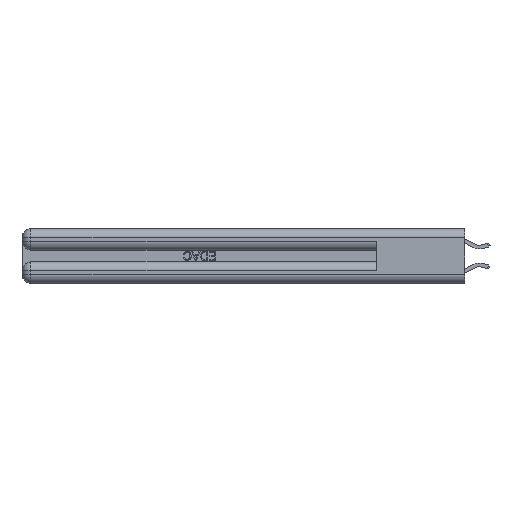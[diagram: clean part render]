
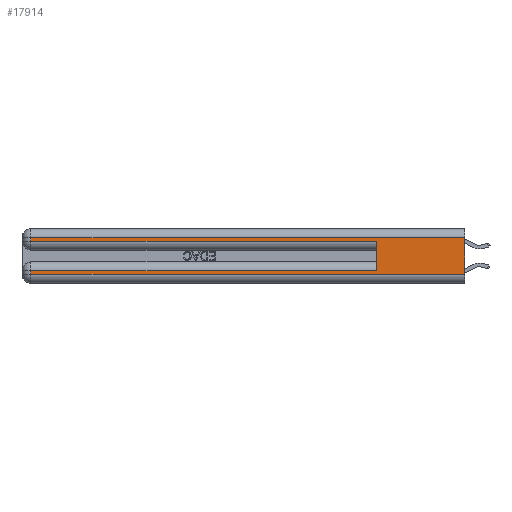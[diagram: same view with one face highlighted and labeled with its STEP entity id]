
A CAD part, left-side view. The second image highlights one B-rep face of the part: STEP entity #17914.
In plain terms, the highlighted planar face has unit normal (-1, 0, 0).
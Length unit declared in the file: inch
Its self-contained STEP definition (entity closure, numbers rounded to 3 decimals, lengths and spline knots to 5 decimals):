
#242 = VERTEX_POINT ( 'NONE', #15075 ) ;
#942 = CARTESIAN_POINT ( 'NONE',  ( 0., 0., 0.06 ) ) ;
#944 = EDGE_CURVE ( 'NONE', #242, #6256, #5850, .T. ) ;
#1041 = FACE_OUTER_BOUND ( 'NONE', #23048, .T. ) ;
#1250 = PLANE ( 'NONE',  #2903 ) ;
#1401 = CARTESIAN_POINT ( 'NONE',  ( 0., 0., 0.37 ) ) ;
#1502 = EDGE_CURVE ( 'NONE', #28715, #6095, #22812, .T. ) ;
#2055 = LINE ( 'NONE', #942, #10357 ) ;
#2480 = CARTESIAN_POINT ( 'NONE',  ( 0., 0.6, 0.285 ) ) ;
#2903 = AXIS2_PLACEMENT_3D ( 'NONE', #13322, #5729, #13222 ) ;
#3819 = DIRECTION ( 'NONE',  ( 0., -1., 0. ) ) ;
#4041 = VECTOR ( 'NONE', #26148, 39.37008 ) ;
#4274 = VERTEX_POINT ( 'NONE', #15329 ) ;
#5330 = CARTESIAN_POINT ( 'NONE',  ( 0., 2.94, 0.37 ) ) ;
#5620 = VECTOR ( 'NONE', #29505, 39.37008 ) ;
#5729 = DIRECTION ( 'NONE',  ( 1., 0., 0. ) ) ;
#5850 = LINE ( 'NONE', #30965, #7732 ) ;
#6095 = VERTEX_POINT ( 'NONE', #23312 ) ;
#6256 = VERTEX_POINT ( 'NONE', #2480 ) ;
#6715 = LINE ( 'NONE', #16120, #9333 ) ;
#6733 = ORIENTED_EDGE ( 'NONE', *, *, #13947, .T. ) ;
#6896 = DIRECTION ( 'NONE',  ( 0., 0., 1. ) ) ;
#7732 = VECTOR ( 'NONE', #6896, 39.37008 ) ;
#8875 = EDGE_CURVE ( 'NONE', #11177, #24480, #23239, .T. ) ;
#9333 = VECTOR ( 'NONE', #3819, 39.37008 ) ;
#9543 = ORIENTED_EDGE ( 'NONE', *, *, #13460, .T. ) ;
#9712 = ORIENTED_EDGE ( 'NONE', *, *, #8875, .T. ) ;
#10357 = VECTOR ( 'NONE', #10653, 39.37008 ) ;
#10653 = DIRECTION ( 'NONE',  ( 0., -1., 0. ) ) ;
#10895 = ORIENTED_EDGE ( 'NONE', *, *, #18679, .T. ) ;
#11177 = VERTEX_POINT ( 'NONE', #25694 ) ;
#11828 = VECTOR ( 'NONE', #20859, 39.37008 ) ;
#12040 = LINE ( 'NONE', #5330, #5620 ) ;
#12128 = CARTESIAN_POINT ( 'NONE',  ( 0., 2.94, 0.37 ) ) ;
#13222 = DIRECTION ( 'NONE',  ( 0., 0., -1. ) ) ;
#13322 = CARTESIAN_POINT ( 'NONE',  ( 0., 0., 0.37 ) ) ;
#13460 = EDGE_CURVE ( 'NONE', #242, #11177, #23698, .T. ) ;
#13947 = EDGE_CURVE ( 'NONE', #4274, #6256, #6715, .T. ) ;
#15075 = CARTESIAN_POINT ( 'NONE',  ( 0., 0.6, 0.085 ) ) ;
#15324 = EDGE_CURVE ( 'NONE', #28715, #24284, #21452, .T. ) ;
#15329 = CARTESIAN_POINT ( 'NONE',  ( 0., 2.94, 0.285 ) ) ;
#15977 = DIRECTION ( 'NONE',  ( 0., 1., 0. ) ) ;
#16120 = CARTESIAN_POINT ( 'NONE',  ( 0., 0., 0.285 ) ) ;
#16568 = ORIENTED_EDGE ( 'NONE', *, *, #1502, .F. ) ;
#17238 = DIRECTION ( 'NONE',  ( 0., 0., -1. ) ) ;
#17914 = ADVANCED_FACE ( 'NONE', ( #1041 ), #1250, .F. ) ;
#18679 = EDGE_CURVE ( 'NONE', #24284, #4274, #12040, .T. ) ;
#19099 = ORIENTED_EDGE ( 'NONE', *, *, #944, .F. ) ;
#19582 = VECTOR ( 'NONE', #15977, 39.37008 ) ;
#20018 = CARTESIAN_POINT ( 'NONE',  ( 0., 0., 0.31 ) ) ;
#20645 = EDGE_CURVE ( 'NONE', #24480, #6095, #2055, .T. ) ;
#20859 = DIRECTION ( 'NONE',  ( 0., 0., -1. ) ) ;
#21235 = CARTESIAN_POINT ( 'NONE',  ( 0., 2.94, 0.31 ) ) ;
#21452 = LINE ( 'NONE', #20018, #19582 ) ;
#22674 = ORIENTED_EDGE ( 'NONE', *, *, #20645, .T. ) ;
#22812 = LINE ( 'NONE', #1401, #11828 ) ;
#23048 = EDGE_LOOP ( 'NONE', ( #16568, #25604, #10895, #6733, #19099, #9543, #9712, #22674 ) ) ;
#23093 = CARTESIAN_POINT ( 'NONE',  ( 0., 0., 0.31 ) ) ;
#23239 = LINE ( 'NONE', #12128, #29645 ) ;
#23312 = CARTESIAN_POINT ( 'NONE',  ( 0., 0., 0.06 ) ) ;
#23698 = LINE ( 'NONE', #30366, #4041 ) ;
#24284 = VERTEX_POINT ( 'NONE', #21235 ) ;
#24480 = VERTEX_POINT ( 'NONE', #26127 ) ;
#25604 = ORIENTED_EDGE ( 'NONE', *, *, #15324, .T. ) ;
#25694 = CARTESIAN_POINT ( 'NONE',  ( 0., 2.94, 0.085 ) ) ;
#26127 = CARTESIAN_POINT ( 'NONE',  ( 0., 2.94, 0.06 ) ) ;
#26148 = DIRECTION ( 'NONE',  ( 0., 1., 0. ) ) ;
#28715 = VERTEX_POINT ( 'NONE', #23093 ) ;
#29505 = DIRECTION ( 'NONE',  ( 0., 0., -1. ) ) ;
#29645 = VECTOR ( 'NONE', #17238, 39.37008 ) ;
#30366 = CARTESIAN_POINT ( 'NONE',  ( 0., 0., 0.085 ) ) ;
#30965 = CARTESIAN_POINT ( 'NONE',  ( 0., 0.6, 0.145 ) ) ;
